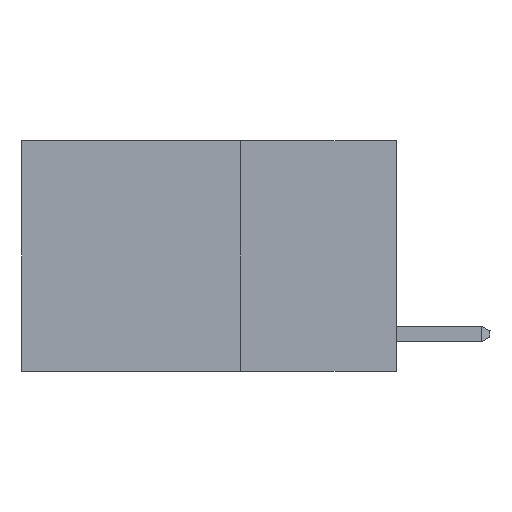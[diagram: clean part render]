
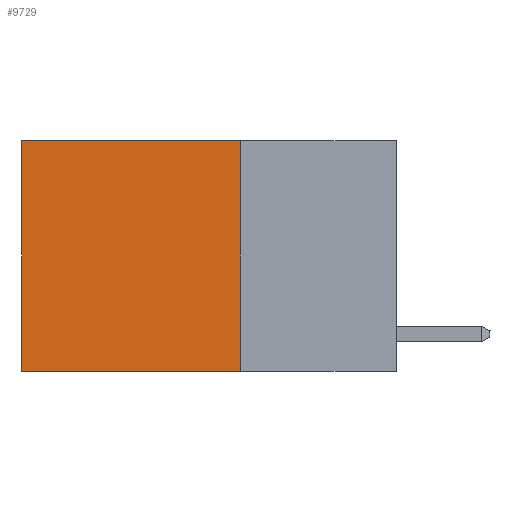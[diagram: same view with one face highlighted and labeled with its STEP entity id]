
A CAD part, left-side view. The second image highlights one B-rep face of the part: STEP entity #9729.
In plain terms, the highlighted planar face has unit normal (-1, 0, 0).
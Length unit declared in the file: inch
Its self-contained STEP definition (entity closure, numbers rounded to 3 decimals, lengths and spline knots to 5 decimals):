
#548 = DIRECTION ( 'NONE',  ( 0., 1., 0. ) ) ;
#890 = DIRECTION ( 'NONE',  ( 0., 0., -1. ) ) ;
#1333 = CARTESIAN_POINT ( 'NONE',  ( 0.2625, 0.25, 0. ) ) ;
#1673 = DIRECTION ( 'NONE',  ( 0., 1., 0. ) ) ;
#2545 = EDGE_CURVE ( 'NONE', #6714, #11514, #2684, .T. ) ;
#2684 = LINE ( 'NONE', #11538, #10695 ) ;
#3494 = VECTOR ( 'NONE', #1673, 39.37008 ) ;
#4162 = DIRECTION ( 'NONE',  ( 1., 0., 0. ) ) ;
#5480 = FACE_OUTER_BOUND ( 'NONE', #13831, .T. ) ;
#5941 = LINE ( 'NONE', #14502, #13955 ) ;
#6048 = DIRECTION ( 'NONE',  ( 0., 0., -1. ) ) ;
#6714 = VERTEX_POINT ( 'NONE', #11963 ) ;
#7362 = LINE ( 'NONE', #16821, #3494 ) ;
#7563 = VECTOR ( 'NONE', #6048, 39.37008 ) ;
#8853 = ORIENTED_EDGE ( 'NONE', *, *, #2545, .T. ) ;
#9729 = ADVANCED_FACE ( 'NONE', ( #5480 ), #13762, .F. ) ;
#10060 = CARTESIAN_POINT ( 'NONE',  ( 0.2625, 0.6, -0.37 ) ) ;
#10159 = AXIS2_PLACEMENT_3D ( 'NONE', #1333, #4162, #12485 ) ;
#10695 = VECTOR ( 'NONE', #548, 39.37008 ) ;
#10858 = VERTEX_POINT ( 'NONE', #10060 ) ;
#11506 = EDGE_CURVE ( 'NONE', #11795, #10858, #7362, .T. ) ;
#11514 = VERTEX_POINT ( 'NONE', #12596 ) ;
#11538 = CARTESIAN_POINT ( 'NONE',  ( 0.2625, 0.25, 0. ) ) ;
#11680 = EDGE_CURVE ( 'NONE', #11514, #10858, #14074, .T. ) ;
#11700 = CARTESIAN_POINT ( 'NONE',  ( 0.2625, 0.6, 0. ) ) ;
#11795 = VERTEX_POINT ( 'NONE', #17667 ) ;
#11963 = CARTESIAN_POINT ( 'NONE',  ( 0.2625, 0.25, 0. ) ) ;
#12350 = ORIENTED_EDGE ( 'NONE', *, *, #11680, .T. ) ;
#12485 = DIRECTION ( 'NONE',  ( 0., 0., -1. ) ) ;
#12596 = CARTESIAN_POINT ( 'NONE',  ( 0.2625, 0.6, 0. ) ) ;
#13762 = PLANE ( 'NONE',  #10159 ) ;
#13831 = EDGE_LOOP ( 'NONE', ( #12350, #14048, #16745, #8853 ) ) ;
#13955 = VECTOR ( 'NONE', #890, 39.37008 ) ;
#14048 = ORIENTED_EDGE ( 'NONE', *, *, #11506, .F. ) ;
#14074 = LINE ( 'NONE', #11700, #7563 ) ;
#14502 = CARTESIAN_POINT ( 'NONE',  ( 0.2625, 0.25, 0. ) ) ;
#14691 = EDGE_CURVE ( 'NONE', #6714, #11795, #5941, .T. ) ;
#16745 = ORIENTED_EDGE ( 'NONE', *, *, #14691, .F. ) ;
#16821 = CARTESIAN_POINT ( 'NONE',  ( 0.2625, 0.25, -0.37 ) ) ;
#17667 = CARTESIAN_POINT ( 'NONE',  ( 0.2625, 0.25, -0.37 ) ) ;
